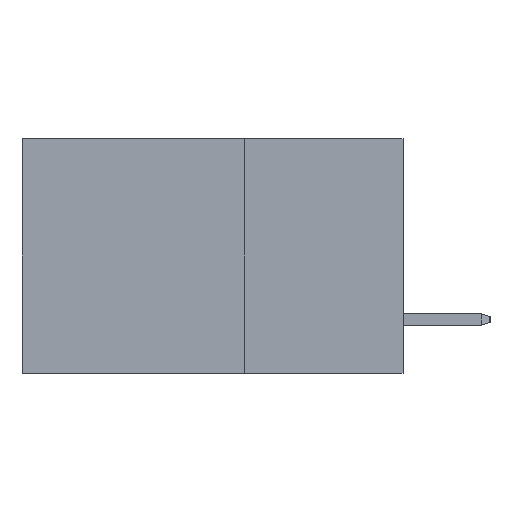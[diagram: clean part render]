
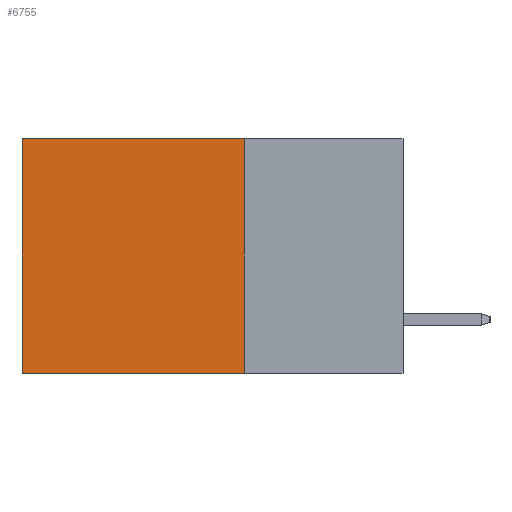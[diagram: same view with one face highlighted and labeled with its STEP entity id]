
A CAD part, left-side view. The second image highlights one B-rep face of the part: STEP entity #6755.
In plain terms, the highlighted planar face has unit normal (-1, 0, 0).
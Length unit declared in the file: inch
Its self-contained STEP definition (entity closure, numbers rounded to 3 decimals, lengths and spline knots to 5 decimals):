
#176 = DIRECTION ( 'NONE',  ( 0., 0., -1. ) ) ;
#361 = EDGE_LOOP ( 'NONE', ( #867, #4657, #3035, #9041 ) ) ;
#397 = CARTESIAN_POINT ( 'NONE',  ( 0.2875, 0.25, -0.37 ) ) ;
#508 = DIRECTION ( 'NONE',  ( 0., 0., -1. ) ) ;
#597 = DIRECTION ( 'NONE',  ( 0., 1., 0. ) ) ;
#652 = FACE_OUTER_BOUND ( 'NONE', #361, .T. ) ;
#696 = DIRECTION ( 'NONE',  ( 0., 1., 0. ) ) ;
#867 = ORIENTED_EDGE ( 'NONE', *, *, #6226, .T. ) ;
#1288 = EDGE_CURVE ( 'NONE', #5709, #4169, #8440, .T. ) ;
#1410 = LINE ( 'NONE', #4322, #6693 ) ;
#2066 = DIRECTION ( 'NONE',  ( 0., 0., -1. ) ) ;
#2796 = CARTESIAN_POINT ( 'NONE',  ( 0.2875, 0.6, 0. ) ) ;
#3035 = ORIENTED_EDGE ( 'NONE', *, *, #6515, .F. ) ;
#4027 = CARTESIAN_POINT ( 'NONE',  ( 0.2875, 0.6, 0. ) ) ;
#4169 = VERTEX_POINT ( 'NONE', #5543 ) ;
#4322 = CARTESIAN_POINT ( 'NONE',  ( 0.2875, 0.25, 0. ) ) ;
#4329 = VECTOR ( 'NONE', #508, 39.37008 ) ;
#4657 = ORIENTED_EDGE ( 'NONE', *, *, #1288, .F. ) ;
#4794 = VERTEX_POINT ( 'NONE', #4027 ) ;
#5092 = DIRECTION ( 'NONE',  ( 1., 0., 0. ) ) ;
#5543 = CARTESIAN_POINT ( 'NONE',  ( 0.2875, 0.6, -0.37 ) ) ;
#5669 = LINE ( 'NONE', #2796, #4329 ) ;
#5709 = VERTEX_POINT ( 'NONE', #7230 ) ;
#5750 = PLANE ( 'NONE',  #6036 ) ;
#6036 = AXIS2_PLACEMENT_3D ( 'NONE', #8109, #5092, #2066 ) ;
#6226 = EDGE_CURVE ( 'NONE', #4794, #4169, #5669, .T. ) ;
#6425 = CARTESIAN_POINT ( 'NONE',  ( 0.2875, 0.25, 0. ) ) ;
#6515 = EDGE_CURVE ( 'NONE', #6715, #5709, #6913, .T. ) ;
#6693 = VECTOR ( 'NONE', #696, 39.37008 ) ;
#6715 = VERTEX_POINT ( 'NONE', #6425 ) ;
#6723 = CARTESIAN_POINT ( 'NONE',  ( 0.2875, 0.25, 0. ) ) ;
#6755 = ADVANCED_FACE ( 'NONE', ( #652 ), #5750, .F. ) ;
#6913 = LINE ( 'NONE', #6723, #6937 ) ;
#6937 = VECTOR ( 'NONE', #176, 39.37008 ) ;
#7230 = CARTESIAN_POINT ( 'NONE',  ( 0.2875, 0.25, -0.37 ) ) ;
#8089 = VECTOR ( 'NONE', #597, 39.37008 ) ;
#8109 = CARTESIAN_POINT ( 'NONE',  ( 0.2875, 0.25, 0. ) ) ;
#8440 = LINE ( 'NONE', #397, #8089 ) ;
#8717 = EDGE_CURVE ( 'NONE', #6715, #4794, #1410, .T. ) ;
#9041 = ORIENTED_EDGE ( 'NONE', *, *, #8717, .T. ) ;
